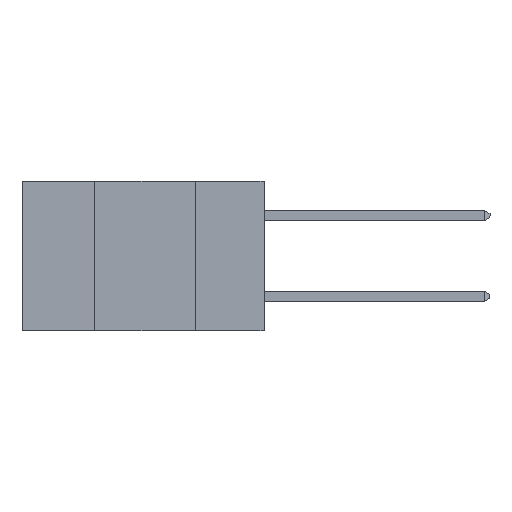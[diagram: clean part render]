
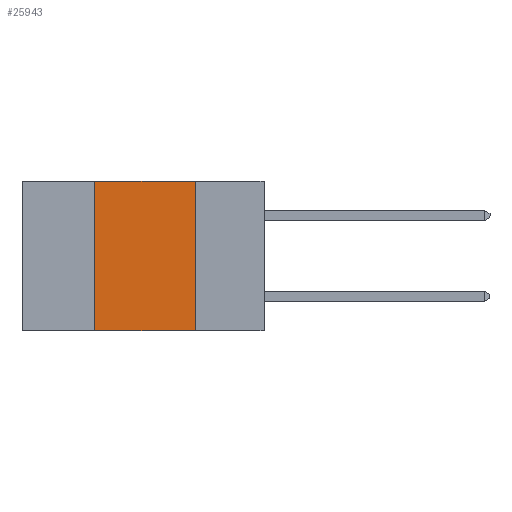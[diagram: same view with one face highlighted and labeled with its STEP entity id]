
A CAD part, left-side view. The second image highlights one B-rep face of the part: STEP entity #25943.
In plain terms, the highlighted planar face has unit normal (-1, 0, 0).
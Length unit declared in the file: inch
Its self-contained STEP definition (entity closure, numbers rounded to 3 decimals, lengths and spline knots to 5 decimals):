
#85 = EDGE_CURVE ( 'NONE', #10093, #7652, #14258, .T. ) ;
#187 = EDGE_CURVE ( 'NONE', #5698, #10093, #27505, .T. ) ;
#977 = DIRECTION ( 'NONE',  ( 0., -1., 0. ) ) ;
#1435 = EDGE_LOOP ( 'NONE', ( #10129, #7779, #2975, #2170 ) ) ;
#2132 = CARTESIAN_POINT ( 'NONE',  ( 0., 0.42, 0. ) ) ;
#2170 = ORIENTED_EDGE ( 'NONE', *, *, #19332, .T. ) ;
#2674 = PLANE ( 'NONE',  #24564 ) ;
#2973 = CARTESIAN_POINT ( 'NONE',  ( 0., 0.17, 0. ) ) ;
#2975 = ORIENTED_EDGE ( 'NONE', *, *, #187, .F. ) ;
#5260 = DIRECTION ( 'NONE',  ( 1., 0., 0. ) ) ;
#5698 = VERTEX_POINT ( 'NONE', #15967 ) ;
#5903 = LINE ( 'NONE', #12404, #31768 ) ;
#7457 = VECTOR ( 'NONE', #31239, 39.37008 ) ;
#7652 = VERTEX_POINT ( 'NONE', #2973 ) ;
#7779 = ORIENTED_EDGE ( 'NONE', *, *, #85, .F. ) ;
#10088 = EDGE_CURVE ( 'NONE', #7652, #25883, #5903, .T. ) ;
#10093 = VERTEX_POINT ( 'NONE', #2132 ) ;
#10129 = ORIENTED_EDGE ( 'NONE', *, *, #10088, .F. ) ;
#10240 = CARTESIAN_POINT ( 'NONE',  ( 0., 0.17, -0.37 ) ) ;
#10350 = CARTESIAN_POINT ( 'NONE',  ( 0., 0.6, 0. ) ) ;
#10931 = VECTOR ( 'NONE', #977, 39.37008 ) ;
#12404 = CARTESIAN_POINT ( 'NONE',  ( 0., 0.17, 0. ) ) ;
#13970 = FACE_OUTER_BOUND ( 'NONE', #1435, .T. ) ;
#14258 = LINE ( 'NONE', #26257, #7457 ) ;
#15967 = CARTESIAN_POINT ( 'NONE',  ( 0., 0.42, -0.37 ) ) ;
#16088 = CARTESIAN_POINT ( 'NONE',  ( 0., 0.42, 0. ) ) ;
#17301 = DIRECTION ( 'NONE',  ( 0., 0., -1. ) ) ;
#18510 = VECTOR ( 'NONE', #27844, 39.37008 ) ;
#19332 = EDGE_CURVE ( 'NONE', #5698, #25883, #23457, .T. ) ;
#22953 = DIRECTION ( 'NONE',  ( 0., 0., -1. ) ) ;
#23457 = LINE ( 'NONE', #31157, #10931 ) ;
#24564 = AXIS2_PLACEMENT_3D ( 'NONE', #10350, #5260, #22953 ) ;
#25883 = VERTEX_POINT ( 'NONE', #10240 ) ;
#25943 = ADVANCED_FACE ( 'NONE', ( #13970 ), #2674, .F. ) ;
#26257 = CARTESIAN_POINT ( 'NONE',  ( 0., 0.6, 0. ) ) ;
#27505 = LINE ( 'NONE', #16088, #18510 ) ;
#27844 = DIRECTION ( 'NONE',  ( 0., 0., 1. ) ) ;
#31157 = CARTESIAN_POINT ( 'NONE',  ( 0., 0.6, -0.37 ) ) ;
#31239 = DIRECTION ( 'NONE',  ( 0., -1., 0. ) ) ;
#31768 = VECTOR ( 'NONE', #17301, 39.37008 ) ;
